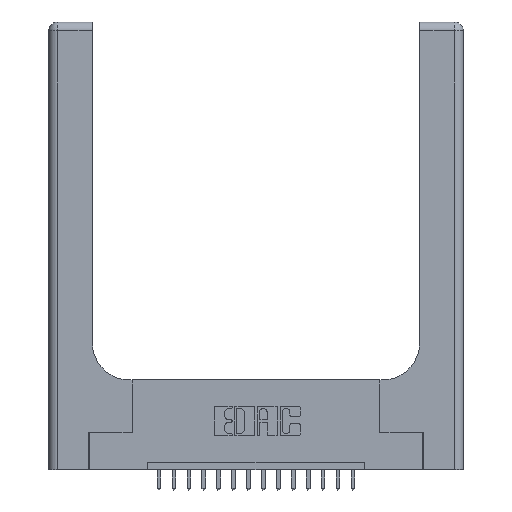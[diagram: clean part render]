
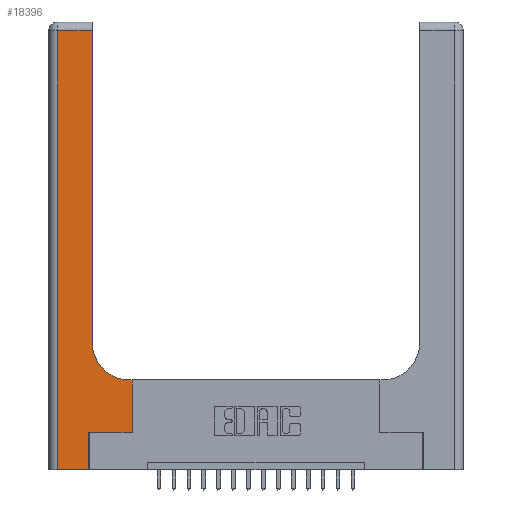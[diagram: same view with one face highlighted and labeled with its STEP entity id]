
A CAD part, top view. The second image highlights one B-rep face of the part: STEP entity #18396.
In plain terms, the highlighted planar face has unit normal (0, 0, 1).
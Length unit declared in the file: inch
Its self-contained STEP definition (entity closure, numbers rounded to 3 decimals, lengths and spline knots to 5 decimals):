
#47 = ORIENTED_EDGE ( 'NONE', *, *, #1918, .T. ) ;
#224 = LINE ( 'NONE', #14521, #5629 ) ;
#307 = ORIENTED_EDGE ( 'NONE', *, *, #12050, .T. ) ;
#345 = EDGE_CURVE ( 'NONE', #7785, #1705, #2253, .T. ) ;
#370 = CARTESIAN_POINT ( 'NONE',  ( 0.5585, 0.25, 0.37 ) ) ;
#1084 = CARTESIAN_POINT ( 'NONE',  ( 0.5415, 0.85, 0.37 ) ) ;
#1124 = LINE ( 'NONE', #5396, #3515 ) ;
#1550 = CARTESIAN_POINT ( 'NONE',  ( 0.269, 0., 0.37 ) ) ;
#1705 = VERTEX_POINT ( 'NONE', #10908 ) ;
#1712 = ORIENTED_EDGE ( 'NONE', *, *, #19323, .T. ) ;
#1771 = EDGE_CURVE ( 'NONE', #17233, #4678, #8153, .T. ) ;
#1868 = ORIENTED_EDGE ( 'NONE', *, *, #10784, .T. ) ;
#1918 = EDGE_CURVE ( 'NONE', #5565, #19267, #17037, .T. ) ;
#1945 = ORIENTED_EDGE ( 'NONE', *, *, #18952, .T. ) ;
#2221 = CARTESIAN_POINT ( 'NONE',  ( 0.269, 0., 0.37 ) ) ;
#2253 = LINE ( 'NONE', #11742, #5789 ) ;
#2887 = DIRECTION ( 'NONE',  ( 0., 1., 0. ) ) ;
#3013 = LINE ( 'NONE', #12269, #3270 ) ;
#3031 = LINE ( 'NONE', #15245, #9673 ) ;
#3228 = DIRECTION ( 'NONE',  ( 1., 0., 0. ) ) ;
#3270 = VECTOR ( 'NONE', #3228, 39.37008 ) ;
#3303 = FACE_OUTER_BOUND ( 'NONE', #11238, .T. ) ;
#3427 = DIRECTION ( 'NONE',  ( 0., 0., -1. ) ) ;
#3515 = VECTOR ( 'NONE', #5456, 39.37008 ) ;
#3921 = CARTESIAN_POINT ( 'NONE',  ( 0.06, 0., 0.37 ) ) ;
#4067 = DIRECTION ( 'NONE',  ( 1., 0., 0. ) ) ;
#4470 = AXIS2_PLACEMENT_3D ( 'NONE', #1084, #11660, #4067 ) ;
#4678 = VERTEX_POINT ( 'NONE', #370 ) ;
#4868 = CARTESIAN_POINT ( 'NONE',  ( 0.5585, 0.6, 0.37 ) ) ;
#5053 = CARTESIAN_POINT ( 'NONE',  ( 0.269, 0.25, 0.37 ) ) ;
#5092 = ORIENTED_EDGE ( 'NONE', *, *, #11106, .T. ) ;
#5396 = CARTESIAN_POINT ( 'NONE',  ( 0., 2.94, 0.37 ) ) ;
#5456 = DIRECTION ( 'NONE',  ( -1., 0., 0. ) ) ;
#5509 = ORIENTED_EDGE ( 'NONE', *, *, #1771, .T. ) ;
#5565 = VERTEX_POINT ( 'NONE', #16210 ) ;
#5629 = VECTOR ( 'NONE', #17591, 39.37008 ) ;
#5789 = VECTOR ( 'NONE', #2887, 39.37008 ) ;
#6375 = ORIENTED_EDGE ( 'NONE', *, *, #9075, .T. ) ;
#7316 = ORIENTED_EDGE ( 'NONE', *, *, #345, .T. ) ;
#7644 = DIRECTION ( 'NONE',  ( -1., 0., 0. ) ) ;
#7752 = VERTEX_POINT ( 'NONE', #1550 ) ;
#7785 = VERTEX_POINT ( 'NONE', #10571 ) ;
#8153 = LINE ( 'NONE', #5053, #12851 ) ;
#8266 = CARTESIAN_POINT ( 'NONE',  ( 0.06, 3., 0.37 ) ) ;
#8618 = VECTOR ( 'NONE', #18724, 39.37008 ) ;
#9075 = EDGE_CURVE ( 'NONE', #7752, #17233, #9975, .T. ) ;
#9636 = CARTESIAN_POINT ( 'NONE',  ( 0.269, 0.25, 0.37 ) ) ;
#9673 = VECTOR ( 'NONE', #7644, 39.37008 ) ;
#9975 = LINE ( 'NONE', #2221, #10443 ) ;
#10005 = VERTEX_POINT ( 'NONE', #4868 ) ;
#10443 = VECTOR ( 'NONE', #15657, 39.37008 ) ;
#10571 = CARTESIAN_POINT ( 'NONE',  ( 0.2915, 0.85, 0.37 ) ) ;
#10784 = EDGE_CURVE ( 'NONE', #1705, #5565, #1124, .T. ) ;
#10908 = CARTESIAN_POINT ( 'NONE',  ( 0.2915, 2.94, 0.37 ) ) ;
#11106 = EDGE_CURVE ( 'NONE', #19267, #7752, #3013, .T. ) ;
#11155 = CARTESIAN_POINT ( 'NONE',  ( 0., 3., 0.37 ) ) ;
#11238 = EDGE_LOOP ( 'NONE', ( #7316, #1868, #47, #5092, #6375, #5509, #1712, #1945, #307 ) ) ;
#11660 = DIRECTION ( 'NONE',  ( 0., 0., -1. ) ) ;
#11742 = CARTESIAN_POINT ( 'NONE',  ( 0.2915, 3., 0.37 ) ) ;
#12050 = EDGE_CURVE ( 'NONE', #16925, #7785, #14432, .T. ) ;
#12269 = CARTESIAN_POINT ( 'NONE',  ( 0., 0., 0.37 ) ) ;
#12789 = AXIS2_PLACEMENT_3D ( 'NONE', #11155, #3427, #18534 ) ;
#12851 = VECTOR ( 'NONE', #15509, 39.37008 ) ;
#14432 = CIRCLE ( 'NONE', #4470, 0.25 ) ;
#14521 = CARTESIAN_POINT ( 'NONE',  ( 0.5585, 0.25, 0.37 ) ) ;
#14889 = CARTESIAN_POINT ( 'NONE',  ( 0.5415, 0.6, 0.37 ) ) ;
#15245 = CARTESIAN_POINT ( 'NONE',  ( 0.2915, 0.6, 0.37 ) ) ;
#15509 = DIRECTION ( 'NONE',  ( 1., 0., 0. ) ) ;
#15657 = DIRECTION ( 'NONE',  ( 0., 1., 0. ) ) ;
#16210 = CARTESIAN_POINT ( 'NONE',  ( 0.06, 2.94, 0.37 ) ) ;
#16925 = VERTEX_POINT ( 'NONE', #14889 ) ;
#16969 = PLANE ( 'NONE',  #12789 ) ;
#17037 = LINE ( 'NONE', #8266, #8618 ) ;
#17233 = VERTEX_POINT ( 'NONE', #9636 ) ;
#17591 = DIRECTION ( 'NONE',  ( 0., 1., 0. ) ) ;
#18396 = ADVANCED_FACE ( 'NONE', ( #3303 ), #16969, .F. ) ;
#18534 = DIRECTION ( 'NONE',  ( -1., 0., 0. ) ) ;
#18724 = DIRECTION ( 'NONE',  ( 0., -1., 0. ) ) ;
#18952 = EDGE_CURVE ( 'NONE', #10005, #16925, #3031, .T. ) ;
#19267 = VERTEX_POINT ( 'NONE', #3921 ) ;
#19323 = EDGE_CURVE ( 'NONE', #4678, #10005, #224, .T. ) ;
